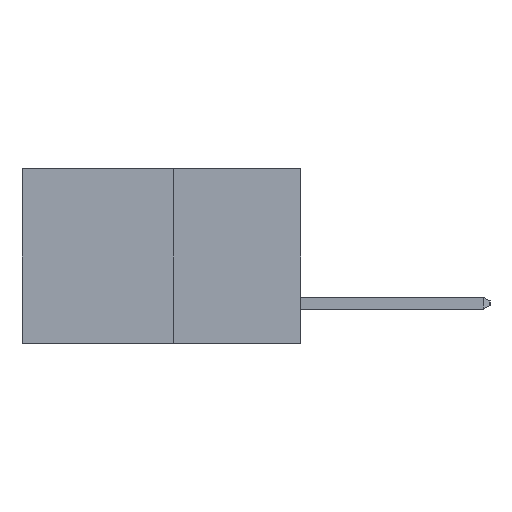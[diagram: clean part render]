
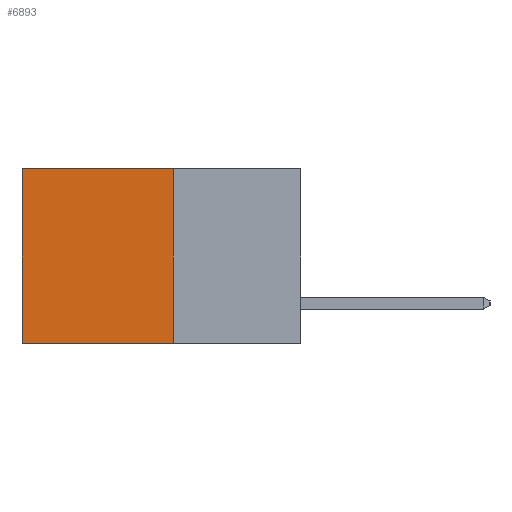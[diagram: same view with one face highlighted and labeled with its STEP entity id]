
A CAD part, left-side view. The second image highlights one B-rep face of the part: STEP entity #6893.
In plain terms, the highlighted planar face has unit normal (-1, 0, 0).
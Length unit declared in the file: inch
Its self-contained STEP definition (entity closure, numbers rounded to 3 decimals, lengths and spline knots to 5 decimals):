
#1146 = ORIENTED_EDGE ( 'NONE', *, *, #11213, .T. ) ;
#1264 = VECTOR ( 'NONE', #3818, 39.37008 ) ;
#1437 = ORIENTED_EDGE ( 'NONE', *, *, #11276, .T. ) ;
#1468 = CARTESIAN_POINT ( 'NONE',  ( 0.277, 0.27, -0.37 ) ) ;
#3012 = DIRECTION ( 'NONE',  ( 0., 1., 0. ) ) ;
#3125 = VERTEX_POINT ( 'NONE', #8459 ) ;
#3169 = EDGE_CURVE ( 'NONE', #9154, #6540, #6243, .T. ) ;
#3778 = VECTOR ( 'NONE', #3012, 39.37008 ) ;
#3818 = DIRECTION ( 'NONE',  ( 0., 0., -1. ) ) ;
#4018 = PLANE ( 'NONE',  #5028 ) ;
#4027 = CARTESIAN_POINT ( 'NONE',  ( 0.277, 0.59, -0.37 ) ) ;
#4101 = VECTOR ( 'NONE', #9862, 39.37008 ) ;
#4698 = CARTESIAN_POINT ( 'NONE',  ( 0.277, 0.27, -0.37 ) ) ;
#4746 = EDGE_LOOP ( 'NONE', ( #1437, #10664, #6131, #1146 ) ) ;
#4909 = EDGE_CURVE ( 'NONE', #10192, #9154, #11413, .T. ) ;
#5028 = AXIS2_PLACEMENT_3D ( 'NONE', #4698, #6740, #7012 ) ;
#6131 = ORIENTED_EDGE ( 'NONE', *, *, #4909, .F. ) ;
#6243 = LINE ( 'NONE', #9233, #3778 ) ;
#6540 = VERTEX_POINT ( 'NONE', #4027 ) ;
#6740 = DIRECTION ( 'NONE',  ( 1., 0., 0. ) ) ;
#6893 = ADVANCED_FACE ( 'NONE', ( #8161 ), #4018, .F. ) ;
#7012 = DIRECTION ( 'NONE',  ( 0., 0., -1. ) ) ;
#7575 = CARTESIAN_POINT ( 'NONE',  ( 0.277, 0.27, 0. ) ) ;
#8161 = FACE_OUTER_BOUND ( 'NONE', #4746, .T. ) ;
#8459 = CARTESIAN_POINT ( 'NONE',  ( 0.277, 0.59, 0. ) ) ;
#8575 = LINE ( 'NONE', #11587, #1264 ) ;
#8981 = CARTESIAN_POINT ( 'NONE',  ( 0.277, 0.27, -0.37 ) ) ;
#9039 = CARTESIAN_POINT ( 'NONE',  ( 0.277, 0.27, 0. ) ) ;
#9154 = VERTEX_POINT ( 'NONE', #1468 ) ;
#9233 = CARTESIAN_POINT ( 'NONE',  ( 0.277, 0.27, -0.37 ) ) ;
#9628 = DIRECTION ( 'NONE',  ( 0., 0., -1. ) ) ;
#9862 = DIRECTION ( 'NONE',  ( 0., 1., 0. ) ) ;
#10192 = VERTEX_POINT ( 'NONE', #7575 ) ;
#10664 = ORIENTED_EDGE ( 'NONE', *, *, #3169, .F. ) ;
#11017 = LINE ( 'NONE', #9039, #4101 ) ;
#11154 = VECTOR ( 'NONE', #9628, 39.37008 ) ;
#11213 = EDGE_CURVE ( 'NONE', #10192, #3125, #11017, .T. ) ;
#11276 = EDGE_CURVE ( 'NONE', #3125, #6540, #8575, .T. ) ;
#11413 = LINE ( 'NONE', #8981, #11154 ) ;
#11587 = CARTESIAN_POINT ( 'NONE',  ( 0.277, 0.59, -0.37 ) ) ;
